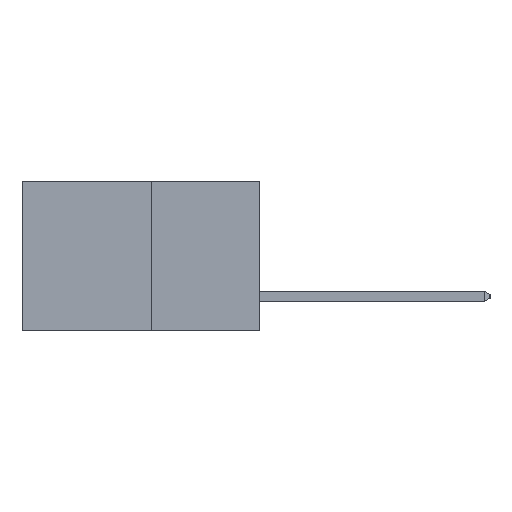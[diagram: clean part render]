
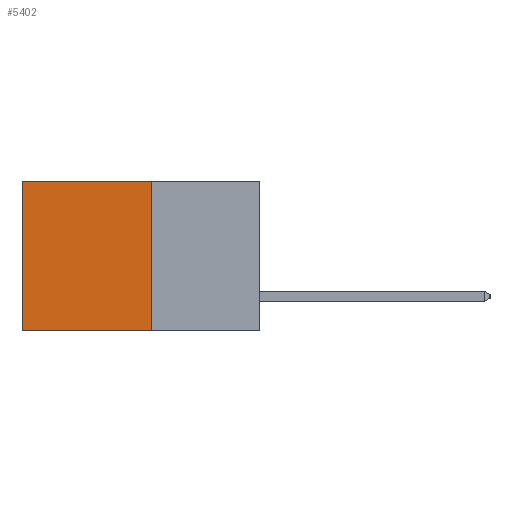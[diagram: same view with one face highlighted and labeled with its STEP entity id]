
A CAD part, left-side view. The second image highlights one B-rep face of the part: STEP entity #5402.
In plain terms, the highlighted planar face has unit normal (-1, 0, 0).
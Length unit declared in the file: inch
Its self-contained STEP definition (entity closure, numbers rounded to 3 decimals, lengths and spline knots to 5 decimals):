
#456 = EDGE_CURVE ( 'NONE', #7797, #16611, #478, .T. ) ;
#478 = LINE ( 'NONE', #5911, #12879 ) ;
#1958 = EDGE_CURVE ( 'NONE', #12584, #2754, #6113, .T. ) ;
#2754 = VERTEX_POINT ( 'NONE', #13414 ) ;
#3058 = DIRECTION ( 'NONE',  ( 0., 0., -1. ) ) ;
#5402 = ADVANCED_FACE ( 'NONE', ( #7639 ), #12176, .F. ) ;
#5630 = VECTOR ( 'NONE', #19113, 39.37008 ) ;
#5911 = CARTESIAN_POINT ( 'NONE',  ( 0.277, 0.59, -0.37 ) ) ;
#6113 = LINE ( 'NONE', #9981, #5630 ) ;
#6647 = LINE ( 'NONE', #8374, #9885 ) ;
#7639 = FACE_OUTER_BOUND ( 'NONE', #12846, .T. ) ;
#7797 = VERTEX_POINT ( 'NONE', #11707 ) ;
#8374 = CARTESIAN_POINT ( 'NONE',  ( 0.277, 0.27, -0.37 ) ) ;
#8682 = VECTOR ( 'NONE', #20291, 39.37008 ) ;
#9509 = CARTESIAN_POINT ( 'NONE',  ( 0.277, 0.59, -0.37 ) ) ;
#9885 = VECTOR ( 'NONE', #19533, 39.37008 ) ;
#9981 = CARTESIAN_POINT ( 'NONE',  ( 0.277, 0.27, -0.37 ) ) ;
#10936 = EDGE_CURVE ( 'NONE', #2754, #16611, #6647, .T. ) ;
#11304 = EDGE_CURVE ( 'NONE', #12584, #7797, #17158, .T. ) ;
#11707 = CARTESIAN_POINT ( 'NONE',  ( 0.277, 0.59, 0. ) ) ;
#12083 = AXIS2_PLACEMENT_3D ( 'NONE', #12246, #12392, #12134 ) ;
#12134 = DIRECTION ( 'NONE',  ( 0., 0., -1. ) ) ;
#12176 = PLANE ( 'NONE',  #12083 ) ;
#12246 = CARTESIAN_POINT ( 'NONE',  ( 0.277, 0.27, -0.37 ) ) ;
#12392 = DIRECTION ( 'NONE',  ( 1., 0., 0. ) ) ;
#12584 = VERTEX_POINT ( 'NONE', #20520 ) ;
#12846 = EDGE_LOOP ( 'NONE', ( #15572, #17054, #19198, #19587 ) ) ;
#12879 = VECTOR ( 'NONE', #3058, 39.37008 ) ;
#13414 = CARTESIAN_POINT ( 'NONE',  ( 0.277, 0.27, -0.37 ) ) ;
#15572 = ORIENTED_EDGE ( 'NONE', *, *, #456, .T. ) ;
#16611 = VERTEX_POINT ( 'NONE', #9509 ) ;
#17054 = ORIENTED_EDGE ( 'NONE', *, *, #10936, .F. ) ;
#17158 = LINE ( 'NONE', #18697, #8682 ) ;
#18697 = CARTESIAN_POINT ( 'NONE',  ( 0.277, 0.27, 0. ) ) ;
#19113 = DIRECTION ( 'NONE',  ( 0., 0., -1. ) ) ;
#19198 = ORIENTED_EDGE ( 'NONE', *, *, #1958, .F. ) ;
#19533 = DIRECTION ( 'NONE',  ( 0., 1., 0. ) ) ;
#19587 = ORIENTED_EDGE ( 'NONE', *, *, #11304, .T. ) ;
#20291 = DIRECTION ( 'NONE',  ( 0., 1., 0. ) ) ;
#20520 = CARTESIAN_POINT ( 'NONE',  ( 0.277, 0.27, 0. ) ) ;
